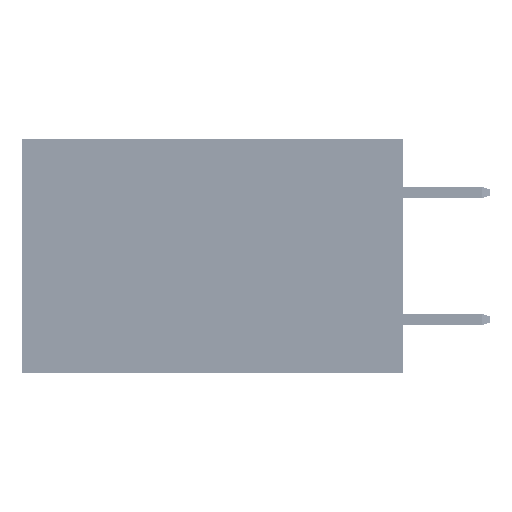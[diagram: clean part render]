
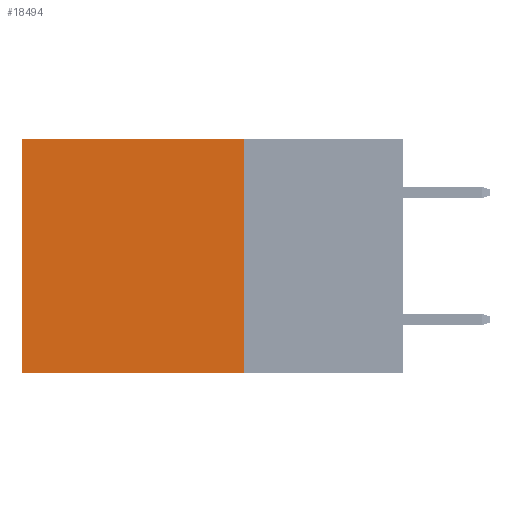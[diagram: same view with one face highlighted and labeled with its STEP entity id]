
A CAD part, left-side view. The second image highlights one B-rep face of the part: STEP entity #18494.
In plain terms, the highlighted planar face has unit normal (-1, 0, 0).
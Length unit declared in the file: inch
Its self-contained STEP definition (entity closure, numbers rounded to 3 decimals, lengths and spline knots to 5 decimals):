
#1060 = VECTOR ( 'NONE', #8601, 39.37008 ) ;
#5316 = DIRECTION ( 'NONE',  ( 1., 0., 0. ) ) ;
#7439 = CARTESIAN_POINT ( 'NONE',  ( 0.2875, 0.6, 0. ) ) ;
#8316 = VERTEX_POINT ( 'NONE', #30268 ) ;
#8578 = CARTESIAN_POINT ( 'NONE',  ( 0.2875, 0.25, -0.37 ) ) ;
#8601 = DIRECTION ( 'NONE',  ( 0., 0., -1. ) ) ;
#8813 = VECTOR ( 'NONE', #30475, 39.37008 ) ;
#9872 = ORIENTED_EDGE ( 'NONE', *, *, #42595, .T. ) ;
#13586 = VERTEX_POINT ( 'NONE', #22190 ) ;
#17595 = EDGE_CURVE ( 'NONE', #34953, #8316, #43833, .T. ) ;
#18494 = ADVANCED_FACE ( 'NONE', ( #19820 ), #42550, .F. ) ;
#19453 = LINE ( 'NONE', #22225, #8813 ) ;
#19820 = FACE_OUTER_BOUND ( 'NONE', #32805, .T. ) ;
#19921 = AXIS2_PLACEMENT_3D ( 'NONE', #35755, #5316, #27607 ) ;
#19989 = ORIENTED_EDGE ( 'NONE', *, *, #28850, .T. ) ;
#20521 = EDGE_CURVE ( 'NONE', #8316, #13586, #32056, .T. ) ;
#20767 = LINE ( 'NONE', #32773, #34103 ) ;
#21524 = DIRECTION ( 'NONE',  ( 0., 0., -1. ) ) ;
#22190 = CARTESIAN_POINT ( 'NONE',  ( 0.2875, 0.6, -0.37 ) ) ;
#22225 = CARTESIAN_POINT ( 'NONE',  ( 0.2875, 0.25, 0. ) ) ;
#24615 = ORIENTED_EDGE ( 'NONE', *, *, #20521, .F. ) ;
#27607 = DIRECTION ( 'NONE',  ( 0., 0., -1. ) ) ;
#28850 = EDGE_CURVE ( 'NONE', #49114, #13586, #20767, .T. ) ;
#30268 = CARTESIAN_POINT ( 'NONE',  ( 0.2875, 0.25, -0.37 ) ) ;
#30475 = DIRECTION ( 'NONE',  ( 0., 1., 0. ) ) ;
#32056 = LINE ( 'NONE', #8578, #41502 ) ;
#32773 = CARTESIAN_POINT ( 'NONE',  ( 0.2875, 0.6, 0. ) ) ;
#32805 = EDGE_LOOP ( 'NONE', ( #19989, #24615, #39212, #9872 ) ) ;
#34103 = VECTOR ( 'NONE', #21524, 39.37008 ) ;
#34953 = VERTEX_POINT ( 'NONE', #38691 ) ;
#35283 = DIRECTION ( 'NONE',  ( 0., 1., 0. ) ) ;
#35755 = CARTESIAN_POINT ( 'NONE',  ( 0.2875, 0.25, 0. ) ) ;
#36338 = CARTESIAN_POINT ( 'NONE',  ( 0.2875, 0.25, 0. ) ) ;
#38691 = CARTESIAN_POINT ( 'NONE',  ( 0.2875, 0.25, 0. ) ) ;
#39212 = ORIENTED_EDGE ( 'NONE', *, *, #17595, .F. ) ;
#41502 = VECTOR ( 'NONE', #35283, 39.37008 ) ;
#42550 = PLANE ( 'NONE',  #19921 ) ;
#42595 = EDGE_CURVE ( 'NONE', #34953, #49114, #19453, .T. ) ;
#43833 = LINE ( 'NONE', #36338, #1060 ) ;
#49114 = VERTEX_POINT ( 'NONE', #7439 ) ;
